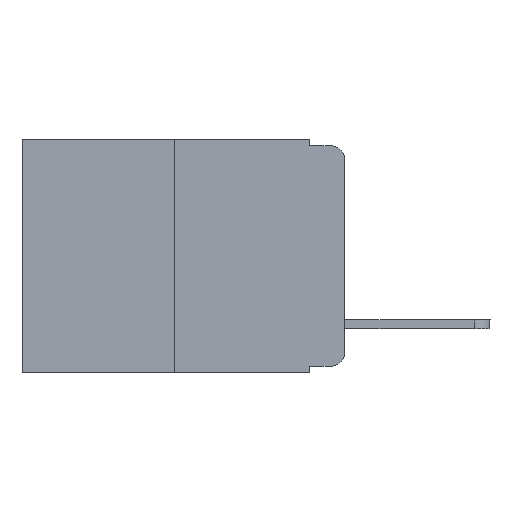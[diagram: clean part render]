
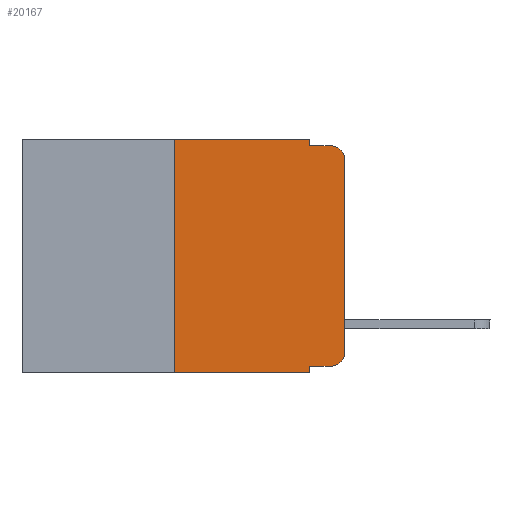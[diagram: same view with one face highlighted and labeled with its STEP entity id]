
A CAD part, left-side view. The second image highlights one B-rep face of the part: STEP entity #20167.
In plain terms, the highlighted planar face has unit normal (-1, 0, 0).
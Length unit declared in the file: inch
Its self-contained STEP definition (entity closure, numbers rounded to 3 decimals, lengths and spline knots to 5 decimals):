
#451 = CARTESIAN_POINT ( 'NONE',  ( 0., 0.25, 0. ) ) ;
#523 = LINE ( 'NONE', #18326, #19821 ) ;
#882 = AXIS2_PLACEMENT_3D ( 'NONE', #15314, #4104, #20664 ) ;
#1100 = ORIENTED_EDGE ( 'NONE', *, *, #10166, .F. ) ;
#1141 = CARTESIAN_POINT ( 'NONE',  ( 0., 0.051, -0.01 ) ) ;
#1360 = VECTOR ( 'NONE', #17411, 39.37008 ) ;
#1570 = LINE ( 'NONE', #20618, #21463 ) ;
#1750 = CIRCLE ( 'NONE', #18632, 0.02 ) ;
#1827 = LINE ( 'NONE', #21468, #9231 ) ;
#2600 = CARTESIAN_POINT ( 'NONE',  ( 0., 0.02, -0.03 ) ) ;
#2852 = CARTESIAN_POINT ( 'NONE',  ( 0., 0.051, 0. ) ) ;
#3098 = CARTESIAN_POINT ( 'NONE',  ( 0., 0.25, -0.343 ) ) ;
#3105 = FACE_OUTER_BOUND ( 'NONE', #11855, .T. ) ;
#3534 = DIRECTION ( 'NONE',  ( 0., 0., -1. ) ) ;
#4104 = DIRECTION ( 'NONE',  ( -1., 0., 0. ) ) ;
#4798 = CARTESIAN_POINT ( 'NONE',  ( 0., 0.473, -0.343 ) ) ;
#5002 = VERTEX_POINT ( 'NONE', #5719 ) ;
#5345 = AXIS2_PLACEMENT_3D ( 'NONE', #21852, #12675, #12751 ) ;
#5699 = VERTEX_POINT ( 'NONE', #9905 ) ;
#5719 = CARTESIAN_POINT ( 'NONE',  ( 0., 0.02, -0.333 ) ) ;
#5867 = VECTOR ( 'NONE', #6622, 39.37008 ) ;
#6140 = EDGE_CURVE ( 'NONE', #5002, #8467, #21120, .T. ) ;
#6476 = VERTEX_POINT ( 'NONE', #12796 ) ;
#6622 = DIRECTION ( 'NONE',  ( 0., -1., 0. ) ) ;
#6937 = VERTEX_POINT ( 'NONE', #2852 ) ;
#7063 = VERTEX_POINT ( 'NONE', #1141 ) ;
#7175 = CARTESIAN_POINT ( 'NONE',  ( 0., 0.051, -0.01 ) ) ;
#7226 = DIRECTION ( 'NONE',  ( 0., 0., -1. ) ) ;
#7492 = CARTESIAN_POINT ( 'NONE',  ( 0., 0., -0.313 ) ) ;
#8351 = EDGE_CURVE ( 'NONE', #7063, #6476, #18067, .T. ) ;
#8371 = VERTEX_POINT ( 'NONE', #22015 ) ;
#8467 = VERTEX_POINT ( 'NONE', #7492 ) ;
#8649 = EDGE_CURVE ( 'NONE', #18640, #5002, #10494, .T. ) ;
#8770 = EDGE_CURVE ( 'NONE', #8371, #6937, #9320, .T. ) ;
#8816 = LINE ( 'NONE', #451, #11424 ) ;
#8999 = DIRECTION ( 'NONE',  ( 0., -1., 0. ) ) ;
#9231 = VECTOR ( 'NONE', #12041, 39.37008 ) ;
#9320 = LINE ( 'NONE', #17485, #20939 ) ;
#9698 = ORIENTED_EDGE ( 'NONE', *, *, #22702, .F. ) ;
#9905 = CARTESIAN_POINT ( 'NONE',  ( 0., 0., -0.03 ) ) ;
#9910 = ORIENTED_EDGE ( 'NONE', *, *, #18971, .F. ) ;
#10166 = EDGE_CURVE ( 'NONE', #6937, #7063, #1570, .T. ) ;
#10290 = LINE ( 'NONE', #4798, #5867 ) ;
#10389 = CARTESIAN_POINT ( 'NONE',  ( 0., 0.051, -0.333 ) ) ;
#10494 = LINE ( 'NONE', #13522, #1360 ) ;
#10928 = DIRECTION ( 'NONE',  ( 0., 0., 1. ) ) ;
#11249 = ORIENTED_EDGE ( 'NONE', *, *, #6140, .T. ) ;
#11424 = VECTOR ( 'NONE', #13571, 39.37008 ) ;
#11855 = EDGE_LOOP ( 'NONE', ( #16398, #18576, #12859, #1100, #20001, #9910, #21697, #9698, #16671, #11249 ) ) ;
#12041 = DIRECTION ( 'NONE',  ( 0., 0., -1. ) ) ;
#12675 = DIRECTION ( 'NONE',  ( 1., 0., 0. ) ) ;
#12751 = DIRECTION ( 'NONE',  ( 0., 0., -1. ) ) ;
#12796 = CARTESIAN_POINT ( 'NONE',  ( 0., 0.02, -0.01 ) ) ;
#12837 = EDGE_CURVE ( 'NONE', #23643, #20481, #10290, .T. ) ;
#12859 = ORIENTED_EDGE ( 'NONE', *, *, #8351, .F. ) ;
#13522 = CARTESIAN_POINT ( 'NONE',  ( 0., 0.051, -0.333 ) ) ;
#13571 = DIRECTION ( 'NONE',  ( 0., 0., 1. ) ) ;
#13682 = CARTESIAN_POINT ( 'NONE',  ( 0., 0.051, -0.343 ) ) ;
#14100 = EDGE_CURVE ( 'NONE', #8467, #5699, #523, .T. ) ;
#15314 = CARTESIAN_POINT ( 'NONE',  ( 0., 0.02, -0.313 ) ) ;
#16227 = PLANE ( 'NONE',  #5345 ) ;
#16398 = ORIENTED_EDGE ( 'NONE', *, *, #14100, .T. ) ;
#16671 = ORIENTED_EDGE ( 'NONE', *, *, #8649, .T. ) ;
#17411 = DIRECTION ( 'NONE',  ( 0., -1., 0. ) ) ;
#17485 = CARTESIAN_POINT ( 'NONE',  ( 0., 0.473, 0. ) ) ;
#18067 = LINE ( 'NONE', #7175, #20668 ) ;
#18126 = EDGE_CURVE ( 'NONE', #5699, #6476, #1750, .T. ) ;
#18326 = CARTESIAN_POINT ( 'NONE',  ( 0., 0., 0. ) ) ;
#18576 = ORIENTED_EDGE ( 'NONE', *, *, #18126, .T. ) ;
#18632 = AXIS2_PLACEMENT_3D ( 'NONE', #2600, #22382, #7226 ) ;
#18640 = VERTEX_POINT ( 'NONE', #10389 ) ;
#18971 = EDGE_CURVE ( 'NONE', #23643, #8371, #8816, .T. ) ;
#19686 = DIRECTION ( 'NONE',  ( 0., -1., 0. ) ) ;
#19821 = VECTOR ( 'NONE', #10928, 39.37008 ) ;
#20001 = ORIENTED_EDGE ( 'NONE', *, *, #8770, .F. ) ;
#20167 = ADVANCED_FACE ( 'NONE', ( #3105 ), #16227, .F. ) ;
#20481 = VERTEX_POINT ( 'NONE', #13682 ) ;
#20618 = CARTESIAN_POINT ( 'NONE',  ( 0., 0.051, 0. ) ) ;
#20664 = DIRECTION ( 'NONE',  ( 0., 0., -1. ) ) ;
#20668 = VECTOR ( 'NONE', #8999, 39.37008 ) ;
#20939 = VECTOR ( 'NONE', #19686, 39.37008 ) ;
#21120 = CIRCLE ( 'NONE', #882, 0.02 ) ;
#21463 = VECTOR ( 'NONE', #3534, 39.37008 ) ;
#21468 = CARTESIAN_POINT ( 'NONE',  ( 0., 0.051, 0. ) ) ;
#21697 = ORIENTED_EDGE ( 'NONE', *, *, #12837, .T. ) ;
#21852 = CARTESIAN_POINT ( 'NONE',  ( 0., 0.473, 0. ) ) ;
#22015 = CARTESIAN_POINT ( 'NONE',  ( 0., 0.25, 0. ) ) ;
#22382 = DIRECTION ( 'NONE',  ( -1., 0., 0. ) ) ;
#22702 = EDGE_CURVE ( 'NONE', #18640, #20481, #1827, .T. ) ;
#23643 = VERTEX_POINT ( 'NONE', #3098 ) ;
